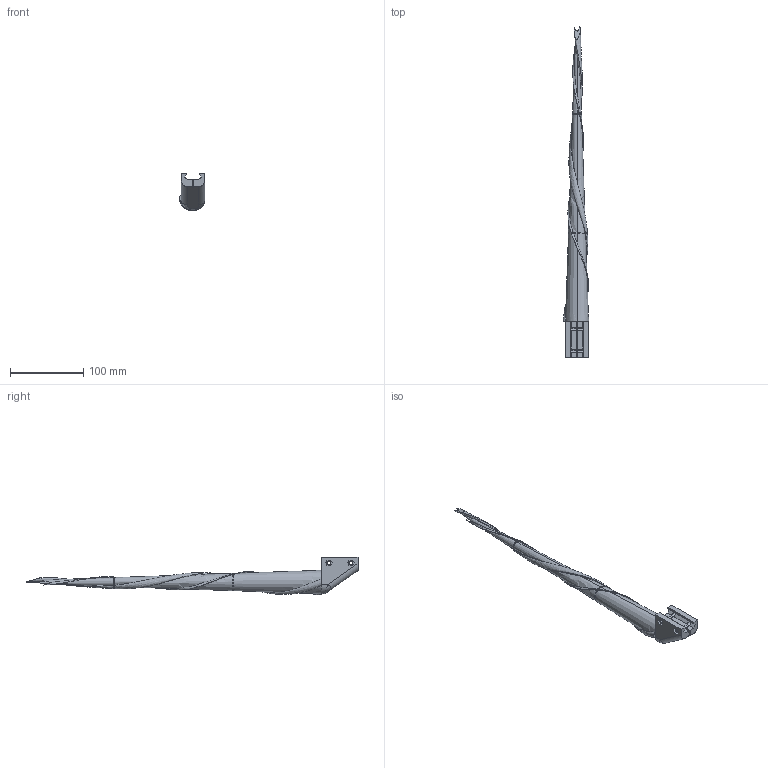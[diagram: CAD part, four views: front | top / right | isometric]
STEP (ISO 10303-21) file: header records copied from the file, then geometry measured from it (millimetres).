
FILE_DESCRIPTION (( 'STEP AP214' ), '1' );
FILE_NAME ('Narwhal.STEP', '2020-05-01T17:25:35', ( '' ), ( '' ), 'SwSTEP 2.0', 'SolidWorks 2019', '' );
FILE_SCHEMA (( 'AUTOMOTIVE_DESIGN' ));
Length unit declared in the file: millimetre
Products named in the file (1): Narwhal
Bounding box: 34.73 x 452.5 x 51.5 mm (x, y, z)
Volume: 169615.3 mm3; surface area: 40141.3 mm2
Topology: 3 solids, 3 shells, 107 faces, 287 edges, 184 vertices
Faces by surface type: plane 55, cone 18, cylinder 17, bspline 17
Entity records: 11515 total; most frequent: CARTESIAN_POINT 9021, ORIENTED_EDGE 574, DIRECTION 428, EDGE_CURVE 287, VERTEX_POINT 184, LINE 146, VECTOR 146, AXIS2_PLACEMENT_3D 141
